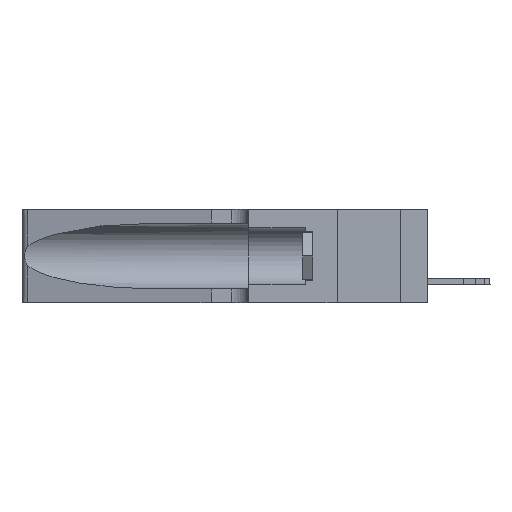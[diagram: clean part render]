
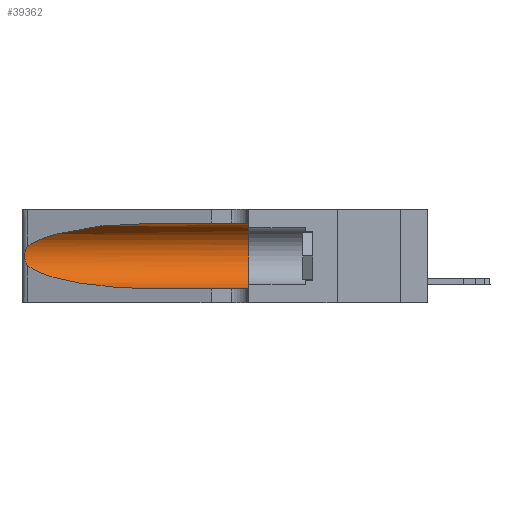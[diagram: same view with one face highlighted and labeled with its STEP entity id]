
A CAD part, left-side view. The second image highlights one B-rep face of the part: STEP entity #39362.
In plain terms, the highlighted cylindrical face has radius 3.308 mm (diameter 6.617 mm), a partial arc.
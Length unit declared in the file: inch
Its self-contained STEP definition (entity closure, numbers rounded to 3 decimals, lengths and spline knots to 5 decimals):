
#1776 = CARTESIAN_POINT ( 'NONE',  ( 0.1305, 1.61858, 0.31525 ) ) ;
#1833 = DIRECTION ( 'NONE',  ( 0., 1., 0. ) ) ;
#2098 = CARTESIAN_POINT ( 'NONE',  ( 0.26018, 1.23835, 0.19895 ) ) ;
#2730 = ORIENTED_EDGE ( 'NONE', *, *, #15799, .T. ) ;
#2969 = VERTEX_POINT ( 'NONE', #4691 ) ;
#3054 = B_SPLINE_CURVE_WITH_KNOTS ( 'NONE', 3,
 ( #23479, #26300, #26565, #8124, #20526, #2098, #23618, #5202, #26699, #39865, #24173, #30212, #12001, #17713 ),
 .UNSPECIFIED., .F., .F.,
 ( 4, 2, 2, 2, 2, 2, 4 ),
 ( 0., 0.00027, 0.00053, 0.00107, 0.0016, 0.00187, 0.00214 ),
 .UNSPECIFIED. ) ;
#3901 = CIRCLE ( 'NONE', #5591, 0.13025 ) ;
#4691 = CARTESIAN_POINT ( 'NONE',  ( 0.1305, 0.72297, 0.31525 ) ) ;
#5202 = CARTESIAN_POINT ( 'NONE',  ( 0.26075, 1.23896, 0.178 ) ) ;
#5215 = CARTESIAN_POINT ( 'NONE',  ( 0.25487, 1.22718, 0.14631 ) ) ;
#5591 = AXIS2_PLACEMENT_3D ( 'NONE', #34960, #1833, #36187 ) ;
#6873 = ORIENTED_EDGE ( 'NONE', *, *, #27163, .T. ) ;
#8048 = CARTESIAN_POINT ( 'NONE',  ( 0.1305, 0.35, 0.31525 ) ) ;
#8124 = CARTESIAN_POINT ( 'NONE',  ( 0.25787, 1.23484, 0.2124 ) ) ;
#8339 = DIRECTION ( 'NONE',  ( 0., -1., 0. ) ) ;
#10611 =( BOUNDED_CURVE ( )  B_SPLINE_CURVE ( 3, ( #5215, #36338, #29818, #26583 ),
 .UNSPECIFIED., .F., .F. ) 
 B_SPLINE_CURVE_WITH_KNOTS ( ( 4, 4 ),
 ( 3.44316, 4.71239 ),
 .UNSPECIFIED. ) 
 CURVE ( )  GEOMETRIC_REPRESENTATION_ITEM ( )  RATIONAL_B_SPLINE_CURVE ( ( 1., 0.87, 0.87, 1. ) ) 
 REPRESENTATION_ITEM ( '' )  );
#10727 = CARTESIAN_POINT ( 'NONE',  ( 0.18966, 0.96281, 0.31525 ) ) ;
#12001 = CARTESIAN_POINT ( 'NONE',  ( 0.25555, 1.22993, 0.14849 ) ) ;
#13451 = CARTESIAN_POINT ( 'NONE',  ( 0.1305, 0.35, 0.05475 ) ) ;
#14280 = CARTESIAN_POINT ( 'NONE',  ( 0.1305, 1.61858, 0.05475 ) ) ;
#14583 = EDGE_CURVE ( 'NONE', #16465, #31113, #3901, .T. ) ;
#15726 = VECTOR ( 'NONE', #8339, 39.37008 ) ;
#15799 = EDGE_CURVE ( 'NONE', #2969, #16038, #31640, .T. ) ;
#16038 = VERTEX_POINT ( 'NONE', #17968 ) ;
#16465 = VERTEX_POINT ( 'NONE', #8048 ) ;
#16997 = DIRECTION ( 'NONE',  ( 0., 0., -1. ) ) ;
#17597 = ORIENTED_EDGE ( 'NONE', *, *, #14583, .F. ) ;
#17713 = CARTESIAN_POINT ( 'NONE',  ( 0.25487, 1.22718, 0.14631 ) ) ;
#17968 = CARTESIAN_POINT ( 'NONE',  ( 0.25487, 1.22718, 0.22369 ) ) ;
#20526 = CARTESIAN_POINT ( 'NONE',  ( 0.25854, 1.2359, 0.20912 ) ) ;
#20856 = EDGE_CURVE ( 'NONE', #2969, #16465, #23954, .T. ) ;
#21762 = AXIS2_PLACEMENT_3D ( 'NONE', #38316, #34909, #16997 ) ;
#22617 = CARTESIAN_POINT ( 'NONE',  ( 0.25487, 1.22718, 0.14631 ) ) ;
#23021 = CARTESIAN_POINT ( 'NONE',  ( 0.1305, 0.72297, 0.31525 ) ) ;
#23455 = DIRECTION ( 'NONE',  ( 0., -1., 0. ) ) ;
#23479 = CARTESIAN_POINT ( 'NONE',  ( 0.25487, 1.22718, 0.22369 ) ) ;
#23618 = CARTESIAN_POINT ( 'NONE',  ( 0.26075, 1.23896, 0.19203 ) ) ;
#23954 = LINE ( 'NONE', #1776, #15726 ) ;
#24173 = CARTESIAN_POINT ( 'NONE',  ( 0.25789, 1.23486, 0.15765 ) ) ;
#25648 = VERTEX_POINT ( 'NONE', #28871 ) ;
#26300 = CARTESIAN_POINT ( 'NONE',  ( 0.25555, 1.22994, 0.2215 ) ) ;
#26565 = CARTESIAN_POINT ( 'NONE',  ( 0.25639, 1.23184, 0.21858 ) ) ;
#26583 = CARTESIAN_POINT ( 'NONE',  ( 0.1305, 0.72297, 0.05475 ) ) ;
#26699 = CARTESIAN_POINT ( 'NONE',  ( 0.26017, 1.23833, 0.17102 ) ) ;
#27163 = EDGE_CURVE ( 'NONE', #39858, #25648, #10611, .T. ) ;
#27435 = ORIENTED_EDGE ( 'NONE', *, *, #36411, .T. ) ;
#28192 = EDGE_CURVE ( 'NONE', #25648, #31113, #28647, .T. ) ;
#28647 = LINE ( 'NONE', #14280, #33025 ) ;
#28871 = CARTESIAN_POINT ( 'NONE',  ( 0.1305, 0.72297, 0.05475 ) ) ;
#29818 = CARTESIAN_POINT ( 'NONE',  ( 0.18966, 0.96281, 0.05475 ) ) ;
#30212 = CARTESIAN_POINT ( 'NONE',  ( 0.25639, 1.23186, 0.15144 ) ) ;
#31019 = CYLINDRICAL_SURFACE ( 'NONE', #21762, 0.13025 ) ;
#31113 = VERTEX_POINT ( 'NONE', #13451 ) ;
#31640 =( BOUNDED_CURVE ( )  B_SPLINE_CURVE ( 3, ( #23021, #10727, #32304, #31785 ),
 .UNSPECIFIED., .F., .F. ) 
 B_SPLINE_CURVE_WITH_KNOTS ( ( 4, 4 ),
 ( 1.5708, 2.84003 ),
 .UNSPECIFIED. ) 
 CURVE ( )  GEOMETRIC_REPRESENTATION_ITEM ( )  RATIONAL_B_SPLINE_CURVE ( ( 1., 0.87, 0.87, 1. ) ) 
 REPRESENTATION_ITEM ( '' )  );
#31785 = CARTESIAN_POINT ( 'NONE',  ( 0.25487, 1.22718, 0.22369 ) ) ;
#32304 = CARTESIAN_POINT ( 'NONE',  ( 0.2373, 1.15595, 0.28018 ) ) ;
#32805 = ORIENTED_EDGE ( 'NONE', *, *, #20856, .F. ) ;
#32981 = FACE_OUTER_BOUND ( 'NONE', #37353, .T. ) ;
#33025 = VECTOR ( 'NONE', #23455, 39.37008 ) ;
#34700 = ORIENTED_EDGE ( 'NONE', *, *, #28192, .T. ) ;
#34909 = DIRECTION ( 'NONE',  ( 0., -1., 0. ) ) ;
#34960 = CARTESIAN_POINT ( 'NONE',  ( 0.1305, 0.35, 0.185 ) ) ;
#36187 = DIRECTION ( 'NONE',  ( 0., 0., 1. ) ) ;
#36338 = CARTESIAN_POINT ( 'NONE',  ( 0.2373, 1.15595, 0.08982 ) ) ;
#36411 = EDGE_CURVE ( 'NONE', #16038, #39858, #3054, .T. ) ;
#37353 = EDGE_LOOP ( 'NONE', ( #2730, #27435, #6873, #34700, #17597, #32805 ) ) ;
#38316 = CARTESIAN_POINT ( 'NONE',  ( 0.1305, 1.61858, 0.185 ) ) ;
#39362 = ADVANCED_FACE ( 'NONE', ( #32981 ), #31019, .F. ) ;
#39858 = VERTEX_POINT ( 'NONE', #22617 ) ;
#39865 = CARTESIAN_POINT ( 'NONE',  ( 0.25856, 1.23593, 0.16098 ) ) ;
